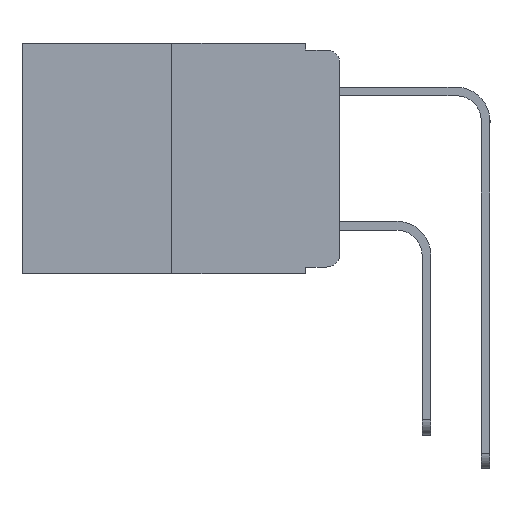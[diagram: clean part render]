
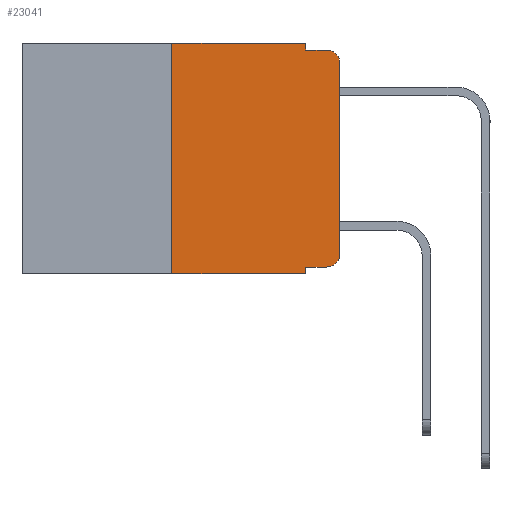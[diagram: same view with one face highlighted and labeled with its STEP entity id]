
A CAD part, left-side view. The second image highlights one B-rep face of the part: STEP entity #23041.
In plain terms, the highlighted planar face has unit normal (-1, 0, 0).
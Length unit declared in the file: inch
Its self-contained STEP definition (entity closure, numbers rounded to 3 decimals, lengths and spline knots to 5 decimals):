
#5 = ORIENTED_EDGE ( 'NONE', *, *, #23491, .F. ) ;
#241 = LINE ( 'NONE', #13272, #10198 ) ;
#242 = CARTESIAN_POINT ( 'NONE',  ( 0., 0.25, 0. ) ) ;
#243 = ORIENTED_EDGE ( 'NONE', *, *, #8090, .F. ) ;
#282 = EDGE_CURVE ( 'NONE', #11317, #11801, #15013, .T. ) ;
#314 = ORIENTED_EDGE ( 'NONE', *, *, #20331, .F. ) ;
#527 = ORIENTED_EDGE ( 'NONE', *, *, #11869, .T. ) ;
#636 = ORIENTED_EDGE ( 'NONE', *, *, #6483, .F. ) ;
#733 = EDGE_CURVE ( 'NONE', #20050, #11317, #9260, .T. ) ;
#879 = FACE_OUTER_BOUND ( 'NONE', #2740, .T. ) ;
#881 = ORIENTED_EDGE ( 'NONE', *, *, #8616, .T. ) ;
#978 = ORIENTED_EDGE ( 'NONE', *, *, #733, .T. ) ;
#1314 = CARTESIAN_POINT ( 'NONE',  ( 0., 0.051, 0. ) ) ;
#1610 = VERTEX_POINT ( 'NONE', #8088 ) ;
#2298 = VERTEX_POINT ( 'NONE', #23184 ) ;
#2315 = VECTOR ( 'NONE', #15031, 39.37008 ) ;
#2383 = DIRECTION ( 'NONE',  ( 0., 0., -1. ) ) ;
#2395 = CARTESIAN_POINT ( 'NONE',  ( 0., 0.473, -0.343 ) ) ;
#2635 = AXIS2_PLACEMENT_3D ( 'NONE', #20850, #4832, #17325 ) ;
#2740 = EDGE_LOOP ( 'NONE', ( #17287, #17502, #20468, #5, #243, #314, #527, #636, #881, #978 ) ) ;
#2798 = VECTOR ( 'NONE', #22059, 39.37008 ) ;
#4188 = CARTESIAN_POINT ( 'NONE',  ( 0., 0.02, -0.313 ) ) ;
#4490 = LINE ( 'NONE', #1314, #13488 ) ;
#4767 = DIRECTION ( 'NONE',  ( -1., 0., 0. ) ) ;
#4832 = DIRECTION ( 'NONE',  ( 1., 0., 0. ) ) ;
#5648 = VERTEX_POINT ( 'NONE', #18536 ) ;
#5770 = LINE ( 'NONE', #15173, #14118 ) ;
#6326 = LINE ( 'NONE', #242, #16301 ) ;
#6355 = CARTESIAN_POINT ( 'NONE',  ( 0., 0.051, -0.343 ) ) ;
#6483 = EDGE_CURVE ( 'NONE', #16015, #18106, #4490, .T. ) ;
#7197 = DIRECTION ( 'NONE',  ( 0., 0., 1. ) ) ;
#7749 = LINE ( 'NONE', #9669, #2798 ) ;
#8088 = CARTESIAN_POINT ( 'NONE',  ( 0., 0.02, -0.01 ) ) ;
#8090 = EDGE_CURVE ( 'NONE', #8509, #20503, #5770, .T. ) ;
#8509 = VERTEX_POINT ( 'NONE', #12785 ) ;
#8616 = EDGE_CURVE ( 'NONE', #16015, #20050, #7749, .T. ) ;
#9260 = CIRCLE ( 'NONE', #20254, 0.02 ) ;
#9641 = CARTESIAN_POINT ( 'NONE',  ( 0., 0.02, -0.03 ) ) ;
#9655 = DIRECTION ( 'NONE',  ( 0., -1., 0. ) ) ;
#9669 = CARTESIAN_POINT ( 'NONE',  ( 0., 0.051, -0.333 ) ) ;
#9914 = VECTOR ( 'NONE', #9655, 39.37008 ) ;
#10198 = VECTOR ( 'NONE', #2383, 39.37008 ) ;
#11181 = EDGE_CURVE ( 'NONE', #2298, #1610, #22928, .T. ) ;
#11317 = VERTEX_POINT ( 'NONE', #22286 ) ;
#11423 = DIRECTION ( 'NONE',  ( 0., 0., -1. ) ) ;
#11513 = LINE ( 'NONE', #2395, #2315 ) ;
#11801 = VERTEX_POINT ( 'NONE', #22022 ) ;
#11869 = EDGE_CURVE ( 'NONE', #5648, #18106, #11513, .T. ) ;
#12102 = CARTESIAN_POINT ( 'NONE',  ( 0., 0., 0. ) ) ;
#12785 = CARTESIAN_POINT ( 'NONE',  ( 0., 0.25, 0. ) ) ;
#13074 = AXIS2_PLACEMENT_3D ( 'NONE', #9641, #22037, #11423 ) ;
#13272 = CARTESIAN_POINT ( 'NONE',  ( 0., 0.051, 0. ) ) ;
#13488 = VECTOR ( 'NONE', #17640, 39.37008 ) ;
#14118 = VECTOR ( 'NONE', #16967, 39.37008 ) ;
#15013 = LINE ( 'NONE', #12102, #18664 ) ;
#15031 = DIRECTION ( 'NONE',  ( 0., -1., 0. ) ) ;
#15173 = CARTESIAN_POINT ( 'NONE',  ( 0., 0.473, 0. ) ) ;
#15357 = CARTESIAN_POINT ( 'NONE',  ( 0., 0.051, -0.333 ) ) ;
#15514 = PLANE ( 'NONE',  #2635 ) ;
#15845 = EDGE_CURVE ( 'NONE', #11801, #1610, #19648, .T. ) ;
#16015 = VERTEX_POINT ( 'NONE', #15357 ) ;
#16301 = VECTOR ( 'NONE', #16628, 39.37008 ) ;
#16628 = DIRECTION ( 'NONE',  ( 0., 0., 1. ) ) ;
#16967 = DIRECTION ( 'NONE',  ( 0., -1., 0. ) ) ;
#17287 = ORIENTED_EDGE ( 'NONE', *, *, #282, .T. ) ;
#17325 = DIRECTION ( 'NONE',  ( 0., 0., -1. ) ) ;
#17502 = ORIENTED_EDGE ( 'NONE', *, *, #15845, .T. ) ;
#17598 = CARTESIAN_POINT ( 'NONE',  ( 0., 0.02, -0.333 ) ) ;
#17640 = DIRECTION ( 'NONE',  ( 0., 0., -1. ) ) ;
#18106 = VERTEX_POINT ( 'NONE', #6355 ) ;
#18536 = CARTESIAN_POINT ( 'NONE',  ( 0., 0.25, -0.343 ) ) ;
#18664 = VECTOR ( 'NONE', #7197, 39.37008 ) ;
#19648 = CIRCLE ( 'NONE', #13074, 0.02 ) ;
#20050 = VERTEX_POINT ( 'NONE', #17598 ) ;
#20218 = CARTESIAN_POINT ( 'NONE',  ( 0., 0.051, -0.01 ) ) ;
#20254 = AXIS2_PLACEMENT_3D ( 'NONE', #4188, #4767, #21189 ) ;
#20331 = EDGE_CURVE ( 'NONE', #5648, #8509, #6326, .T. ) ;
#20468 = ORIENTED_EDGE ( 'NONE', *, *, #11181, .F. ) ;
#20503 = VERTEX_POINT ( 'NONE', #20706 ) ;
#20706 = CARTESIAN_POINT ( 'NONE',  ( 0., 0.051, 0. ) ) ;
#20850 = CARTESIAN_POINT ( 'NONE',  ( 0., 0.473, 0. ) ) ;
#21189 = DIRECTION ( 'NONE',  ( 0., 0., -1. ) ) ;
#22022 = CARTESIAN_POINT ( 'NONE',  ( 0., 0., -0.03 ) ) ;
#22037 = DIRECTION ( 'NONE',  ( -1., 0., 0. ) ) ;
#22059 = DIRECTION ( 'NONE',  ( 0., -1., 0. ) ) ;
#22286 = CARTESIAN_POINT ( 'NONE',  ( 0., 0., -0.313 ) ) ;
#22928 = LINE ( 'NONE', #20218, #9914 ) ;
#23041 = ADVANCED_FACE ( 'NONE', ( #879 ), #15514, .F. ) ;
#23184 = CARTESIAN_POINT ( 'NONE',  ( 0., 0.051, -0.01 ) ) ;
#23491 = EDGE_CURVE ( 'NONE', #20503, #2298, #241, .T. ) ;
